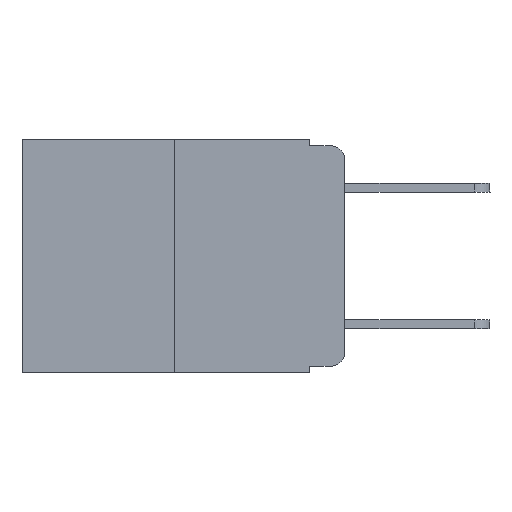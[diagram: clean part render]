
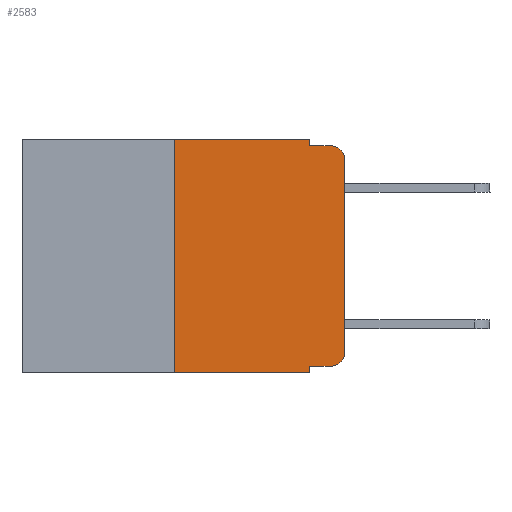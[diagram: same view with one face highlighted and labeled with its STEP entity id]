
A CAD part, left-side view. The second image highlights one B-rep face of the part: STEP entity #2583.
In plain terms, the highlighted planar face has unit normal (-1, 0, 0).
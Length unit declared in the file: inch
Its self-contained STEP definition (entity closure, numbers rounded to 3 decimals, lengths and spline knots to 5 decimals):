
#658 = EDGE_CURVE ( 'NONE', #12576, #15194, #7404, .T. ) ;
#744 = DIRECTION ( 'NONE',  ( 1., 0., 0. ) ) ;
#807 = DIRECTION ( 'NONE',  ( 0., -1., 0. ) ) ;
#1269 = ORIENTED_EDGE ( 'NONE', *, *, #14815, .T. ) ;
#1370 = ORIENTED_EDGE ( 'NONE', *, *, #4930, .F. ) ;
#1383 = ORIENTED_EDGE ( 'NONE', *, *, #11379, .T. ) ;
#1572 = ORIENTED_EDGE ( 'NONE', *, *, #8028, .F. ) ;
#1811 = VERTEX_POINT ( 'NONE', #15986 ) ;
#1896 = FACE_OUTER_BOUND ( 'NONE', #3869, .T. ) ;
#2019 = VECTOR ( 'NONE', #7445, 39.37008 ) ;
#2190 = DIRECTION ( 'NONE',  ( 0., 0., -1. ) ) ;
#2194 = VERTEX_POINT ( 'NONE', #11347 ) ;
#2322 = ORIENTED_EDGE ( 'NONE', *, *, #3455, .T. ) ;
#2364 = VECTOR ( 'NONE', #6086, 39.37008 ) ;
#2583 = ADVANCED_FACE ( 'NONE', ( #1896 ), #14059, .F. ) ;
#2785 = DIRECTION ( 'NONE',  ( 0., 0., -1. ) ) ;
#3169 = CARTESIAN_POINT ( 'NONE',  ( 0., 0.02, -0.313 ) ) ;
#3423 = CARTESIAN_POINT ( 'NONE',  ( 0., 0.02, -0.333 ) ) ;
#3455 = EDGE_CURVE ( 'NONE', #12576, #6732, #5960, .T. ) ;
#3502 = DIRECTION ( 'NONE',  ( 0., -1., 0. ) ) ;
#3517 = VECTOR ( 'NONE', #807, 39.37008 ) ;
#3615 = CARTESIAN_POINT ( 'NONE',  ( 0., 0., 0. ) ) ;
#3688 = AXIS2_PLACEMENT_3D ( 'NONE', #14032, #12607, #16413 ) ;
#3790 = CARTESIAN_POINT ( 'NONE',  ( 0., 0.051, -0.343 ) ) ;
#3869 = EDGE_LOOP ( 'NONE', ( #8550, #1269, #1572, #7288, #12573, #6321, #2322, #1370, #1383, #13539 ) ) ;
#3952 = CARTESIAN_POINT ( 'NONE',  ( 0., 0.051, -0.333 ) ) ;
#4122 = CARTESIAN_POINT ( 'NONE',  ( 0., 0.25, 0. ) ) ;
#4569 = DIRECTION ( 'NONE',  ( 0., -1., 0. ) ) ;
#4788 = CARTESIAN_POINT ( 'NONE',  ( 0., 0.473, 0. ) ) ;
#4930 = EDGE_CURVE ( 'NONE', #8606, #6732, #7894, .T. ) ;
#5960 = LINE ( 'NONE', #12822, #2019 ) ;
#6086 = DIRECTION ( 'NONE',  ( 0., 0., 1. ) ) ;
#6321 = ORIENTED_EDGE ( 'NONE', *, *, #658, .F. ) ;
#6334 = CARTESIAN_POINT ( 'NONE',  ( 0., 0.051, -0.01 ) ) ;
#6607 = VERTEX_POINT ( 'NONE', #7053 ) ;
#6708 = VECTOR ( 'NONE', #2190, 39.37008 ) ;
#6732 = VERTEX_POINT ( 'NONE', #3790 ) ;
#6786 = EDGE_CURVE ( 'NONE', #15368, #2194, #13217, .T. ) ;
#7033 = DIRECTION ( 'NONE',  ( -1., 0., 0. ) ) ;
#7053 = CARTESIAN_POINT ( 'NONE',  ( 0., 0.02, -0.01 ) ) ;
#7288 = ORIENTED_EDGE ( 'NONE', *, *, #12530, .F. ) ;
#7404 = LINE ( 'NONE', #16933, #2364 ) ;
#7445 = DIRECTION ( 'NONE',  ( 0., -1., 0. ) ) ;
#7842 = VECTOR ( 'NONE', #2785, 39.37008 ) ;
#7894 = LINE ( 'NONE', #13272, #7842 ) ;
#7913 = CIRCLE ( 'NONE', #3688, 0.02 ) ;
#8028 = EDGE_CURVE ( 'NONE', #10824, #6607, #9263, .T. ) ;
#8539 = VERTEX_POINT ( 'NONE', #3423 ) ;
#8550 = ORIENTED_EDGE ( 'NONE', *, *, #6786, .T. ) ;
#8606 = VERTEX_POINT ( 'NONE', #3952 ) ;
#8811 = EDGE_CURVE ( 'NONE', #15194, #1811, #13743, .T. ) ;
#9263 = LINE ( 'NONE', #6334, #3517 ) ;
#9693 = VECTOR ( 'NONE', #11719, 39.37008 ) ;
#9948 = CARTESIAN_POINT ( 'NONE',  ( 0., 0., -0.313 ) ) ;
#9966 = CARTESIAN_POINT ( 'NONE',  ( 0., 0.051, 0. ) ) ;
#9973 = DIRECTION ( 'NONE',  ( 0., 0., -1. ) ) ;
#10476 = CIRCLE ( 'NONE', #15801, 0.02 ) ;
#10824 = VERTEX_POINT ( 'NONE', #11799 ) ;
#10904 = VECTOR ( 'NONE', #4569, 39.37008 ) ;
#11104 = CARTESIAN_POINT ( 'NONE',  ( 0., 0.473, 0. ) ) ;
#11347 = CARTESIAN_POINT ( 'NONE',  ( 0., 0., -0.03 ) ) ;
#11379 = EDGE_CURVE ( 'NONE', #8606, #8539, #17251, .T. ) ;
#11719 = DIRECTION ( 'NONE',  ( 0., 0., 1. ) ) ;
#11799 = CARTESIAN_POINT ( 'NONE',  ( 0., 0.051, -0.01 ) ) ;
#12363 = AXIS2_PLACEMENT_3D ( 'NONE', #4788, #744, #12632 ) ;
#12530 = EDGE_CURVE ( 'NONE', #1811, #10824, #16900, .T. ) ;
#12573 = ORIENTED_EDGE ( 'NONE', *, *, #8811, .F. ) ;
#12576 = VERTEX_POINT ( 'NONE', #15925 ) ;
#12607 = DIRECTION ( 'NONE',  ( -1., 0., 0. ) ) ;
#12632 = DIRECTION ( 'NONE',  ( 0., 0., -1. ) ) ;
#12822 = CARTESIAN_POINT ( 'NONE',  ( 0., 0.473, -0.343 ) ) ;
#13217 = LINE ( 'NONE', #3615, #9693 ) ;
#13272 = CARTESIAN_POINT ( 'NONE',  ( 0., 0.051, 0. ) ) ;
#13539 = ORIENTED_EDGE ( 'NONE', *, *, #16576, .T. ) ;
#13743 = LINE ( 'NONE', #11104, #10904 ) ;
#14032 = CARTESIAN_POINT ( 'NONE',  ( 0., 0.02, -0.03 ) ) ;
#14059 = PLANE ( 'NONE',  #12363 ) ;
#14815 = EDGE_CURVE ( 'NONE', #2194, #6607, #7913, .T. ) ;
#15136 = VECTOR ( 'NONE', #3502, 39.37008 ) ;
#15194 = VERTEX_POINT ( 'NONE', #4122 ) ;
#15368 = VERTEX_POINT ( 'NONE', #9948 ) ;
#15801 = AXIS2_PLACEMENT_3D ( 'NONE', #3169, #7033, #9973 ) ;
#15925 = CARTESIAN_POINT ( 'NONE',  ( 0., 0.25, -0.343 ) ) ;
#15986 = CARTESIAN_POINT ( 'NONE',  ( 0., 0.051, 0. ) ) ;
#16413 = DIRECTION ( 'NONE',  ( 0., 0., -1. ) ) ;
#16576 = EDGE_CURVE ( 'NONE', #8539, #15368, #10476, .T. ) ;
#16900 = LINE ( 'NONE', #9966, #6708 ) ;
#16933 = CARTESIAN_POINT ( 'NONE',  ( 0., 0.25, 0. ) ) ;
#17251 = LINE ( 'NONE', #17340, #15136 ) ;
#17340 = CARTESIAN_POINT ( 'NONE',  ( 0., 0.051, -0.333 ) ) ;
